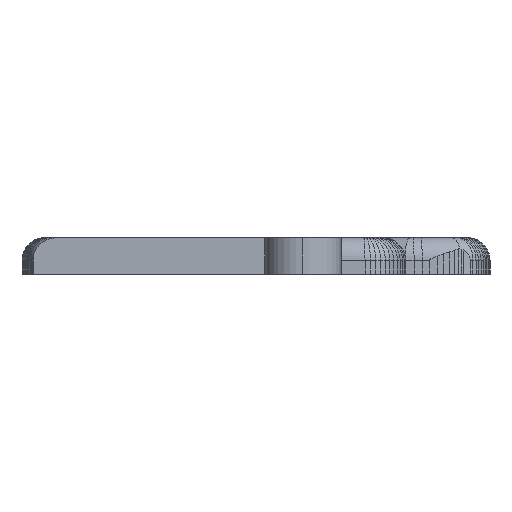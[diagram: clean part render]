
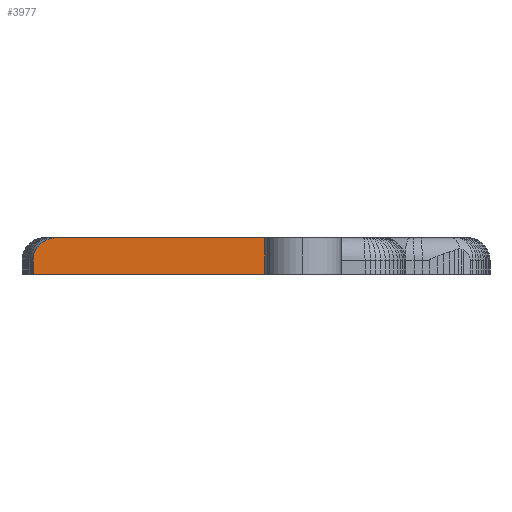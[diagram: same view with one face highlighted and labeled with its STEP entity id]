
A CAD part, left-side view. The second image highlights one B-rep face of the part: STEP entity #3977.
In plain terms, the highlighted planar face has unit normal (-1, 0, 0).
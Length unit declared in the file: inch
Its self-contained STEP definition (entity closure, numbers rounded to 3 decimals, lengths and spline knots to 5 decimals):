
#126 = DIRECTION ( 'NONE',  ( 0., 1., 0. ) ) ;
#232 = CARTESIAN_POINT ( 'NONE',  ( 2.96745, 0.9384, 0.11016 ) ) ;
#346 = VERTEX_POINT ( 'NONE', #3395 ) ;
#1398 = CARTESIAN_POINT ( 'NONE',  ( 2.96745, 0.9384, 0. ) ) ;
#1515 = ORIENTED_EDGE ( 'NONE', *, *, #13221, .F. ) ;
#1822 = CARTESIAN_POINT ( 'NONE',  ( 2.96745, -0.2996, 0.19685 ) ) ;
#1917 = CARTESIAN_POINT ( 'NONE',  ( 2.96745, -0.19256, 0.19685 ) ) ;
#2675 = CARTESIAN_POINT ( 'NONE',  ( 2.96745, 0.81057, 0.19685 ) ) ;
#2785 = CARTESIAN_POINT ( 'NONE',  ( 2.96745, -0.19256, 0. ) ) ;
#2845 = CARTESIAN_POINT ( 'NONE',  ( 2.96745, 0.87165, 0.19685 ) ) ;
#3316 = DIRECTION ( 'NONE',  ( 0., 0., 1. ) ) ;
#3391 = ORIENTED_EDGE ( 'NONE', *, *, #14453, .F. ) ;
#3395 = CARTESIAN_POINT ( 'NONE',  ( 2.96745, 0.9384, 0.11016 ) ) ;
#3636 = CARTESIAN_POINT ( 'NONE',  ( 2.96745, 0.9384, 0. ) ) ;
#3693 = EDGE_LOOP ( 'NONE', ( #13150, #15073, #7864, #3391, #1515 ) ) ;
#3725 = EDGE_CURVE ( 'NONE', #11950, #346, #9958, .T. ) ;
#3778 = EDGE_CURVE ( 'NONE', #16139, #11950, #6134, .T. ) ;
#3956 =( BOUNDED_CURVE ( )  B_SPLINE_CURVE ( 3, ( #232, #13088, #2845, #2675 ),
 .UNSPECIFIED., .F., .F. ) 
 B_SPLINE_CURVE_WITH_KNOTS ( ( 4, 4 ),
 ( 0.29387, 1.5708 ),
 .UNSPECIFIED. ) 
 CURVE ( )  GEOMETRIC_REPRESENTATION_ITEM ( )  RATIONAL_B_SPLINE_CURVE ( ( 1., 0.869, 0.869, 1. ) ) 
 REPRESENTATION_ITEM ( '' )  );
#3977 = ADVANCED_FACE ( 'NONE', ( #16170 ), #14868, .F. ) ;
#5358 = VECTOR ( 'NONE', #10908, 39.37008 ) ;
#5492 = DIRECTION ( 'NONE',  ( 0., 0., -1. ) ) ;
#6134 = LINE ( 'NONE', #2785, #10749 ) ;
#6836 = VERTEX_POINT ( 'NONE', #1822 ) ;
#7864 = ORIENTED_EDGE ( 'NONE', *, *, #12480, .T. ) ;
#8822 = VERTEX_POINT ( 'NONE', #11171 ) ;
#9197 = DIRECTION ( 'NONE',  ( 0., 0., 1. ) ) ;
#9611 = DIRECTION ( 'NONE',  ( 1., 0., 0. ) ) ;
#9662 = CARTESIAN_POINT ( 'NONE',  ( 2.96745, 0.19037, 0. ) ) ;
#9951 = CARTESIAN_POINT ( 'NONE',  ( 2.96745, -0.2996, 0. ) ) ;
#9958 = LINE ( 'NONE', #1398, #10156 ) ;
#10156 = VECTOR ( 'NONE', #9197, 39.37008 ) ;
#10539 = LINE ( 'NONE', #13889, #14350 ) ;
#10749 = VECTOR ( 'NONE', #126, 39.37008 ) ;
#10908 = DIRECTION ( 'NONE',  ( 0., -1., 0. ) ) ;
#11171 = CARTESIAN_POINT ( 'NONE',  ( 2.96745, 0.81057, 0.19685 ) ) ;
#11950 = VERTEX_POINT ( 'NONE', #3636 ) ;
#12480 = EDGE_CURVE ( 'NONE', #16139, #6836, #10539, .T. ) ;
#12986 = LINE ( 'NONE', #1917, #5358 ) ;
#13088 = CARTESIAN_POINT ( 'NONE',  ( 2.96745, 0.92071, 0.16358 ) ) ;
#13150 = ORIENTED_EDGE ( 'NONE', *, *, #3725, .F. ) ;
#13221 = EDGE_CURVE ( 'NONE', #346, #8822, #3956, .T. ) ;
#13889 = CARTESIAN_POINT ( 'NONE',  ( 2.96745, -0.2996, 0.19685 ) ) ;
#14350 = VECTOR ( 'NONE', #3316, 39.37008 ) ;
#14453 = EDGE_CURVE ( 'NONE', #8822, #6836, #12986, .T. ) ;
#14868 = PLANE ( 'NONE',  #15715 ) ;
#15073 = ORIENTED_EDGE ( 'NONE', *, *, #3778, .F. ) ;
#15715 = AXIS2_PLACEMENT_3D ( 'NONE', #9662, #9611, #5492 ) ;
#16139 = VERTEX_POINT ( 'NONE', #9951 ) ;
#16170 = FACE_OUTER_BOUND ( 'NONE', #3693, .T. ) ;
